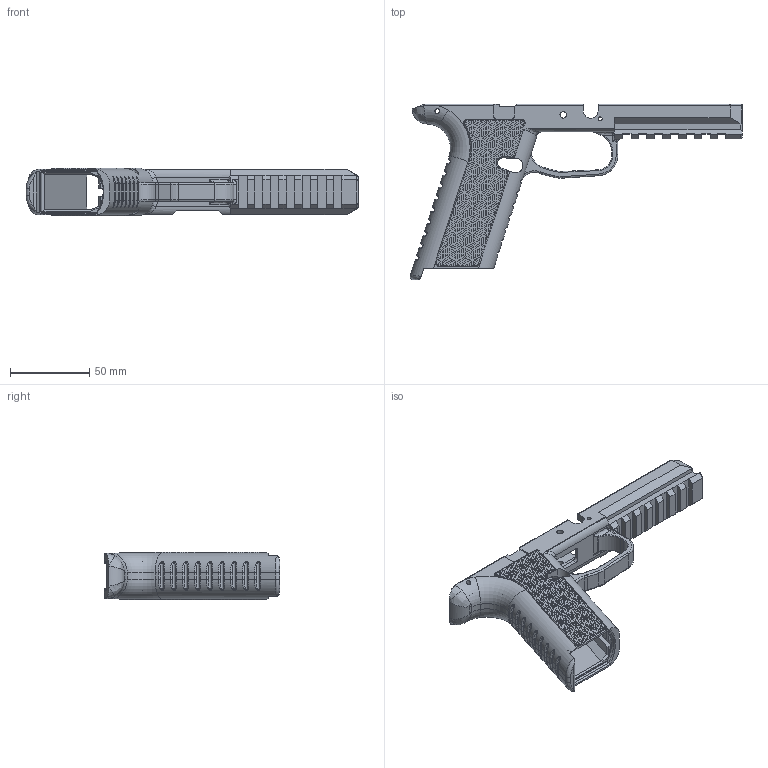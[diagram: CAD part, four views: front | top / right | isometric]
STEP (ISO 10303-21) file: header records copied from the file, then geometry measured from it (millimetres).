
FILE_DESCRIPTION(/* description */ (''),/* implementation_level */ '2;1');
FILE_NAME(/* name */ '40L Frame.step',/* time_stamp */ '2021-07-12T09:02:24-06:00',/* author */ (''),/* organization */ (''),/* preprocessor_version */ 'ST-DEVELOPER v18.1',/* originating_system */ 'Autodesk Translation Framework v10.9.0.1377',/* authorisation */ '');
FILE_SCHEMA (('AUTOMOTIVE_DESIGN { 1 0 10303 214 3 1 1 }'));
Length unit declared in the file: millimetre
Products named in the file (2): FNS Release; Standard Size Grip
Assembly tree (1 placements, depth 2):
  FNS Release
    Standard Size Grip
Bounding box: 209.87 x 110.97 x 30 mm (x, y, z)
Volume: 92724.6 mm3; surface area: 51657.2 mm2
Topology: 1 solids, 1 shells, 4064 faces, 10884 edges, 7102 vertices
Faces by surface type: plane 2252, bspline 1566, cylinder 198, torus 42, cone 6
Full cylindrical faces by diameter (mm): 2.5 x2, 3 x2, 4.1 x2
Entity records: 134298 total; most frequent: CARTESIAN_POINT 47892, ORIENTED_EDGE 21762, DIRECTION 13173, EDGE_CURVE 10881, LINE 7231, VECTOR 7231, VERTEX_POINT 7102, EDGE_LOOP 4369
